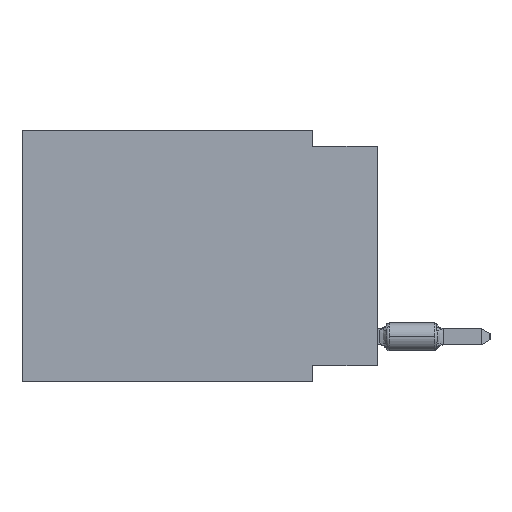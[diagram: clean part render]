
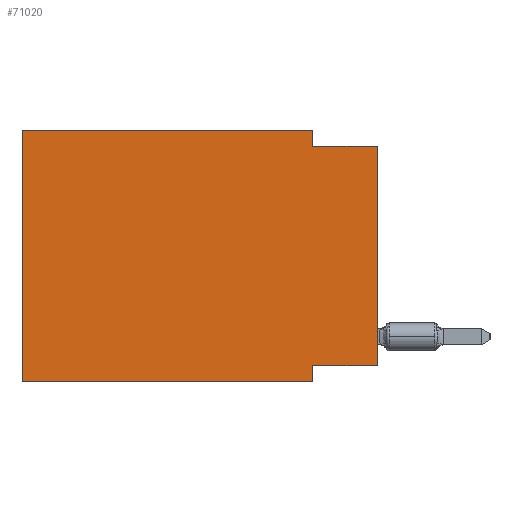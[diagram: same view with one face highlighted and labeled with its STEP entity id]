
A CAD part, left-side view. The second image highlights one B-rep face of the part: STEP entity #71020.
In plain terms, the highlighted planar face has unit normal (-1, 0, 0).
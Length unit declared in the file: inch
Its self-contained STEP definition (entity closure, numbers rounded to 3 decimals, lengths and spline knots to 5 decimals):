
#424 = ORIENTED_EDGE ( 'NONE', *, *, #61554, .F. ) ;
#798 = EDGE_CURVE ( 'NONE', #16457, #52379, #54023, .T. ) ;
#2368 = EDGE_CURVE ( 'NONE', #15433, #37008, #29615, .T. ) ;
#6970 = ORIENTED_EDGE ( 'NONE', *, *, #798, .F. ) ;
#8966 = VERTEX_POINT ( 'NONE', #75343 ) ;
#9016 = EDGE_CURVE ( 'NONE', #34856, #8966, #45680, .T. ) ;
#9354 = CARTESIAN_POINT ( 'NONE',  ( 0., 0., -0.365 ) ) ;
#9800 = VECTOR ( 'NONE', #22620, 39.37008 ) ;
#12227 = VERTEX_POINT ( 'NONE', #37847 ) ;
#12650 = DIRECTION ( 'NONE',  ( 0., 0., -1. ) ) ;
#13406 = DIRECTION ( 'NONE',  ( 0., -1., 0. ) ) ;
#15433 = VERTEX_POINT ( 'NONE', #25577 ) ;
#15696 = DIRECTION ( 'NONE',  ( 0., 0., 1. ) ) ;
#16337 = LINE ( 'NONE', #9354, #74698 ) ;
#16355 = CARTESIAN_POINT ( 'NONE',  ( 0., 0.1, 0. ) ) ;
#16457 = VERTEX_POINT ( 'NONE', #16355 ) ;
#17055 = EDGE_LOOP ( 'NONE', ( #56945, #18197, #6970, #56195, #37970, #54423, #63859, #424 ) ) ;
#17434 = VECTOR ( 'NONE', #12650, 39.37008 ) ;
#17474 = CARTESIAN_POINT ( 'NONE',  ( 0., 0.1, -0.365 ) ) ;
#18197 = ORIENTED_EDGE ( 'NONE', *, *, #49055, .F. ) ;
#18561 = LINE ( 'NONE', #42369, #41872 ) ;
#20189 = CARTESIAN_POINT ( 'NONE',  ( 0., 0.1, -0.025 ) ) ;
#22620 = DIRECTION ( 'NONE',  ( 0., -1., 0. ) ) ;
#23320 = VECTOR ( 'NONE', #25302, 39.37008 ) ;
#25302 = DIRECTION ( 'NONE',  ( 0., -1., 0. ) ) ;
#25577 = CARTESIAN_POINT ( 'NONE',  ( 0., 0., -0.365 ) ) ;
#27672 = DIRECTION ( 'NONE',  ( 0., 1., 0. ) ) ;
#28106 = CARTESIAN_POINT ( 'NONE',  ( 0., 0.55, -0.39 ) ) ;
#29615 = LINE ( 'NONE', #75021, #56522 ) ;
#29871 = DIRECTION ( 'NONE',  ( 0., 0., -1. ) ) ;
#31758 = LINE ( 'NONE', #73130, #38696 ) ;
#34560 = DIRECTION ( 'NONE',  ( 0., 0., 1. ) ) ;
#34856 = VERTEX_POINT ( 'NONE', #58323 ) ;
#35605 = DIRECTION ( 'NONE',  ( 0., 0., -1. ) ) ;
#37008 = VERTEX_POINT ( 'NONE', #70796 ) ;
#37847 = CARTESIAN_POINT ( 'NONE',  ( 0., 0.55, 0. ) ) ;
#37970 = ORIENTED_EDGE ( 'NONE', *, *, #73594, .F. ) ;
#38696 = VECTOR ( 'NONE', #13406, 39.37008 ) ;
#40053 = LINE ( 'NONE', #65392, #66005 ) ;
#41481 = DIRECTION ( 'NONE',  ( 1., 0., 0. ) ) ;
#41824 = AXIS2_PLACEMENT_3D ( 'NONE', #64874, #41481, #35605 ) ;
#41872 = VECTOR ( 'NONE', #34560, 39.37008 ) ;
#42308 = EDGE_CURVE ( 'NONE', #12227, #16457, #31758, .T. ) ;
#42369 = CARTESIAN_POINT ( 'NONE',  ( 0., 0.55, 0. ) ) ;
#45680 = LINE ( 'NONE', #28106, #9800 ) ;
#49055 = EDGE_CURVE ( 'NONE', #52379, #37008, #66267, .T. ) ;
#52379 = VERTEX_POINT ( 'NONE', #20189 ) ;
#54023 = LINE ( 'NONE', #60650, #17434 ) ;
#54423 = ORIENTED_EDGE ( 'NONE', *, *, #9016, .T. ) ;
#56195 = ORIENTED_EDGE ( 'NONE', *, *, #42308, .F. ) ;
#56522 = VECTOR ( 'NONE', #15696, 39.37008 ) ;
#56945 = ORIENTED_EDGE ( 'NONE', *, *, #2368, .T. ) ;
#58323 = CARTESIAN_POINT ( 'NONE',  ( 0., 0.55, -0.39 ) ) ;
#59806 = PLANE ( 'NONE',  #41824 ) ;
#60650 = CARTESIAN_POINT ( 'NONE',  ( 0., 0.1, 0. ) ) ;
#61554 = EDGE_CURVE ( 'NONE', #15433, #70279, #16337, .T. ) ;
#63859 = ORIENTED_EDGE ( 'NONE', *, *, #76103, .F. ) ;
#64874 = CARTESIAN_POINT ( 'NONE',  ( 0., 0.55, 0. ) ) ;
#65392 = CARTESIAN_POINT ( 'NONE',  ( 0., 0.1, -0.39 ) ) ;
#66005 = VECTOR ( 'NONE', #29871, 39.37008 ) ;
#66028 = FACE_OUTER_BOUND ( 'NONE', #17055, .T. ) ;
#66267 = LINE ( 'NONE', #72537, #23320 ) ;
#70279 = VERTEX_POINT ( 'NONE', #17474 ) ;
#70796 = CARTESIAN_POINT ( 'NONE',  ( 0., 0., -0.025 ) ) ;
#71020 = ADVANCED_FACE ( 'NONE', ( #66028 ), #59806, .F. ) ;
#72537 = CARTESIAN_POINT ( 'NONE',  ( 0., 0., -0.025 ) ) ;
#73130 = CARTESIAN_POINT ( 'NONE',  ( 0., 0.55, 0. ) ) ;
#73594 = EDGE_CURVE ( 'NONE', #34856, #12227, #18561, .T. ) ;
#74698 = VECTOR ( 'NONE', #27672, 39.37008 ) ;
#75021 = CARTESIAN_POINT ( 'NONE',  ( 0., 0., 0. ) ) ;
#75343 = CARTESIAN_POINT ( 'NONE',  ( 0., 0.1, -0.39 ) ) ;
#76103 = EDGE_CURVE ( 'NONE', #70279, #8966, #40053, .T. ) ;
